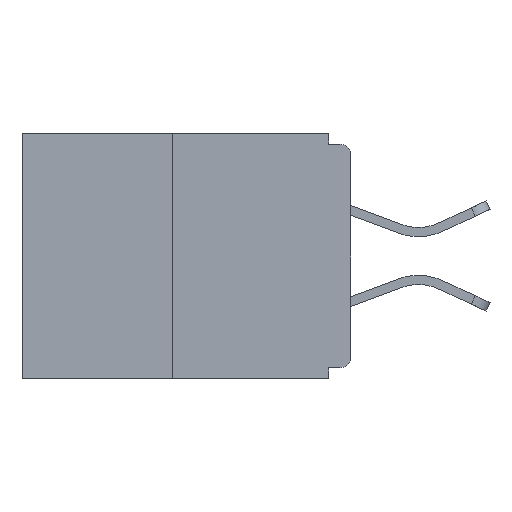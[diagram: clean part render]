
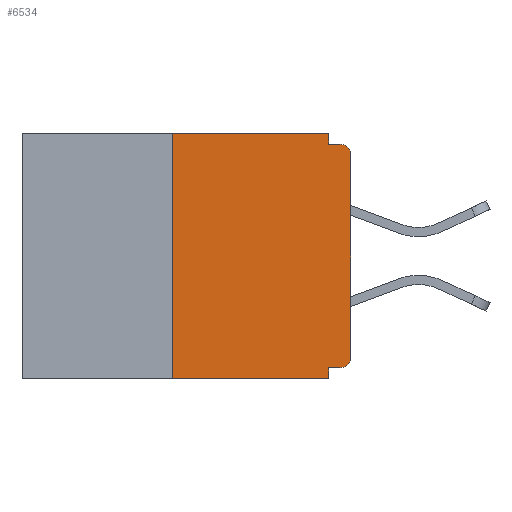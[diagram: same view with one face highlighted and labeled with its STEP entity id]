
A CAD part, left-side view. The second image highlights one B-rep face of the part: STEP entity #6534.
In plain terms, the highlighted planar face has unit normal (-1, 0, 0).
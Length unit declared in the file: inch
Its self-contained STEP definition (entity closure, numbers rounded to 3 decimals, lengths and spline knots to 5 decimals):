
#147 = DIRECTION ( 'NONE',  ( 0., -1., 0. ) ) ;
#295 = LINE ( 'NONE', #6257, #15781 ) ;
#651 = EDGE_CURVE ( 'NONE', #2359, #2117, #10887, .T. ) ;
#1021 = EDGE_CURVE ( 'NONE', #16982, #18641, #19677, .T. ) ;
#1397 = CARTESIAN_POINT ( 'NONE',  ( 0., 0., -0.03 ) ) ;
#1640 = VECTOR ( 'NONE', #3770, 39.37008 ) ;
#1691 = CARTESIAN_POINT ( 'NONE',  ( 0., 0.25, 0. ) ) ;
#2117 = VERTEX_POINT ( 'NONE', #18772 ) ;
#2315 = LINE ( 'NONE', #12761, #13068 ) ;
#2359 = VERTEX_POINT ( 'NONE', #11109 ) ;
#2684 = CARTESIAN_POINT ( 'NONE',  ( 0., 0.031, -0.328 ) ) ;
#2785 = ORIENTED_EDGE ( 'NONE', *, *, #17119, .F. ) ;
#3214 = EDGE_CURVE ( 'NONE', #2359, #11194, #4813, .T. ) ;
#3536 = CARTESIAN_POINT ( 'NONE',  ( 0., 0., -0.328 ) ) ;
#3770 = DIRECTION ( 'NONE',  ( 0., 0., 1. ) ) ;
#3794 = VECTOR ( 'NONE', #6630, 39.37008 ) ;
#3830 = VECTOR ( 'NONE', #17135, 39.37008 ) ;
#3983 = EDGE_CURVE ( 'NONE', #2117, #15739, #16739, .T. ) ;
#4067 = CARTESIAN_POINT ( 'NONE',  ( 0., 0.031, 0. ) ) ;
#4813 = LINE ( 'NONE', #3536, #3794 ) ;
#4822 = ORIENTED_EDGE ( 'NONE', *, *, #14287, .F. ) ;
#4836 = CIRCLE ( 'NONE', #20146, 0.015 ) ;
#4856 = CARTESIAN_POINT ( 'NONE',  ( 0., 0., 0. ) ) ;
#5165 = CARTESIAN_POINT ( 'NONE',  ( 0., 0.25, 0. ) ) ;
#6257 = CARTESIAN_POINT ( 'NONE',  ( 0., 0., -0.015 ) ) ;
#6316 = EDGE_CURVE ( 'NONE', #15739, #16191, #4836, .T. ) ;
#6534 = ADVANCED_FACE ( 'NONE', ( #14020 ), #12780, .F. ) ;
#6630 = DIRECTION ( 'NONE',  ( 0., 1., 0. ) ) ;
#7640 = ORIENTED_EDGE ( 'NONE', *, *, #651, .T. ) ;
#8012 = CARTESIAN_POINT ( 'NONE',  ( 0., 0.031, -0.343 ) ) ;
#8019 = ORIENTED_EDGE ( 'NONE', *, *, #19714, .F. ) ;
#8124 = LINE ( 'NONE', #12243, #3830 ) ;
#8230 = ORIENTED_EDGE ( 'NONE', *, *, #3214, .F. ) ;
#8504 = CARTESIAN_POINT ( 'NONE',  ( 0., 0.015, -0.03 ) ) ;
#8533 = VECTOR ( 'NONE', #11906, 39.37008 ) ;
#8768 = DIRECTION ( 'NONE',  ( 0., 0., -1. ) ) ;
#8769 = VECTOR ( 'NONE', #14174, 39.37008 ) ;
#8802 = AXIS2_PLACEMENT_3D ( 'NONE', #15205, #11881, #11817 ) ;
#9479 = CARTESIAN_POINT ( 'NONE',  ( 0., 0.46, 0. ) ) ;
#10017 = EDGE_CURVE ( 'NONE', #11194, #12240, #8124, .T. ) ;
#10109 = CARTESIAN_POINT ( 'NONE',  ( 0., 0.031, 0. ) ) ;
#10469 = CARTESIAN_POINT ( 'NONE',  ( 0., 0.46, -0.343 ) ) ;
#10776 = DIRECTION ( 'NONE',  ( 0., -1., 0. ) ) ;
#10887 = CIRCLE ( 'NONE', #8802, 0.015 ) ;
#11102 = ORIENTED_EDGE ( 'NONE', *, *, #10017, .F. ) ;
#11106 = VECTOR ( 'NONE', #13722, 39.37008 ) ;
#11109 = CARTESIAN_POINT ( 'NONE',  ( 0., 0.015, -0.328 ) ) ;
#11194 = VERTEX_POINT ( 'NONE', #2684 ) ;
#11497 = ORIENTED_EDGE ( 'NONE', *, *, #6316, .T. ) ;
#11817 = DIRECTION ( 'NONE',  ( 0., 0., -1. ) ) ;
#11881 = DIRECTION ( 'NONE',  ( -1., 0., 0. ) ) ;
#11906 = DIRECTION ( 'NONE',  ( 0., 0., -1. ) ) ;
#12240 = VERTEX_POINT ( 'NONE', #8012 ) ;
#12243 = CARTESIAN_POINT ( 'NONE',  ( 0., 0.031, -0.343 ) ) ;
#12597 = LINE ( 'NONE', #10469, #11106 ) ;
#12652 = DIRECTION ( 'NONE',  ( 0., 0., -1. ) ) ;
#12761 = CARTESIAN_POINT ( 'NONE',  ( 0., 0.46, 0. ) ) ;
#12780 = PLANE ( 'NONE',  #18390 ) ;
#13068 = VECTOR ( 'NONE', #147, 39.37008 ) ;
#13340 = DIRECTION ( 'NONE',  ( -1., 0., 0. ) ) ;
#13722 = DIRECTION ( 'NONE',  ( 0., -1., 0. ) ) ;
#13887 = CARTESIAN_POINT ( 'NONE',  ( 0., 0.015, -0.015 ) ) ;
#14020 = FACE_OUTER_BOUND ( 'NONE', #17729, .T. ) ;
#14174 = DIRECTION ( 'NONE',  ( 0., 0., 1. ) ) ;
#14287 = EDGE_CURVE ( 'NONE', #14816, #16191, #295, .T. ) ;
#14591 = ORIENTED_EDGE ( 'NONE', *, *, #16866, .T. ) ;
#14816 = VERTEX_POINT ( 'NONE', #19800 ) ;
#15205 = CARTESIAN_POINT ( 'NONE',  ( 0., 0.015, -0.313 ) ) ;
#15739 = VERTEX_POINT ( 'NONE', #1397 ) ;
#15781 = VECTOR ( 'NONE', #10776, 39.37008 ) ;
#15935 = ORIENTED_EDGE ( 'NONE', *, *, #1021, .F. ) ;
#16024 = DIRECTION ( 'NONE',  ( 1., 0., 0. ) ) ;
#16191 = VERTEX_POINT ( 'NONE', #13887 ) ;
#16739 = LINE ( 'NONE', #4856, #8769 ) ;
#16866 = EDGE_CURVE ( 'NONE', #16982, #12240, #12597, .T. ) ;
#16982 = VERTEX_POINT ( 'NONE', #18838 ) ;
#17119 = EDGE_CURVE ( 'NONE', #18641, #20336, #2315, .T. ) ;
#17135 = DIRECTION ( 'NONE',  ( 0., 0., -1. ) ) ;
#17729 = EDGE_LOOP ( 'NONE', ( #2785, #15935, #14591, #11102, #8230, #7640, #20032, #11497, #4822, #8019 ) ) ;
#18390 = AXIS2_PLACEMENT_3D ( 'NONE', #9479, #16024, #12652 ) ;
#18641 = VERTEX_POINT ( 'NONE', #5165 ) ;
#18772 = CARTESIAN_POINT ( 'NONE',  ( 0., 0., -0.313 ) ) ;
#18838 = CARTESIAN_POINT ( 'NONE',  ( 0., 0.25, -0.343 ) ) ;
#19677 = LINE ( 'NONE', #1691, #1640 ) ;
#19714 = EDGE_CURVE ( 'NONE', #20336, #14816, #19807, .T. ) ;
#19800 = CARTESIAN_POINT ( 'NONE',  ( 0., 0.031, -0.015 ) ) ;
#19807 = LINE ( 'NONE', #4067, #8533 ) ;
#20032 = ORIENTED_EDGE ( 'NONE', *, *, #3983, .T. ) ;
#20146 = AXIS2_PLACEMENT_3D ( 'NONE', #8504, #13340, #8768 ) ;
#20336 = VERTEX_POINT ( 'NONE', #10109 ) ;
